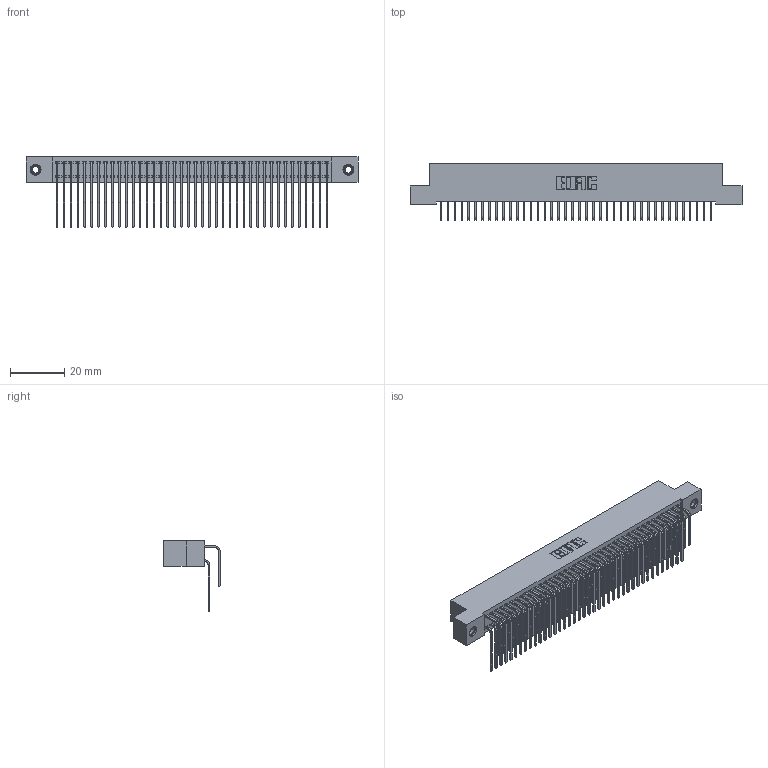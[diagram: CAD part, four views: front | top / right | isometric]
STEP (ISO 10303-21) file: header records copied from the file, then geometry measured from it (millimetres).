
FILE_DESCRIPTION (( 'STEP AP203' ), '1' );
FILE_NAME ('392-080-559-207.STEP', '2018-08-18T03:18:35', ( '' ), ( '' ), 'SwSTEP 2.0', 'SolidWorks 2016', '' );
FILE_SCHEMA (( 'CONFIG_CONTROL_DESIGN' ));
Length unit declared in the file: inch
Products named in the file (5): 342 Part_TI; 345-292-001_558 559 Tail - 1; 345-292-001_559 Tail - 2; 345-250-001_345-250-005-103; 392-080-559-207
Assembly tree (83 placements, depth 2):
  392-080-559-207
    342 Part_TI
    345-292-001_558 559 Tail - 1  x40
    345-292-001_559 Tail - 2  x40
    345-250-001_345-250-005-103  x2
Bounding box: 121.92 x 20.64 x 25.78 mm (x, y, z)
Volume: 11393.8 mm3; surface area: 20610.5 mm2
Topology: 83 solids, 83 shells, 4490 faces, 13315 edges, 8762 vertices
Faces by surface type: plane 3138, cylinder 1336, cone 12, torus 4
Entity records: 28830 total; most frequent: CARTESIAN_POINT 4812, ORIENTED_EDGE 4690, DIRECTION 4127, EDGE_CURVE 2345, VECTOR 2157, LINE 2157, VERTEX_POINT 1556, AXIS2_PLACEMENT_3D 985
